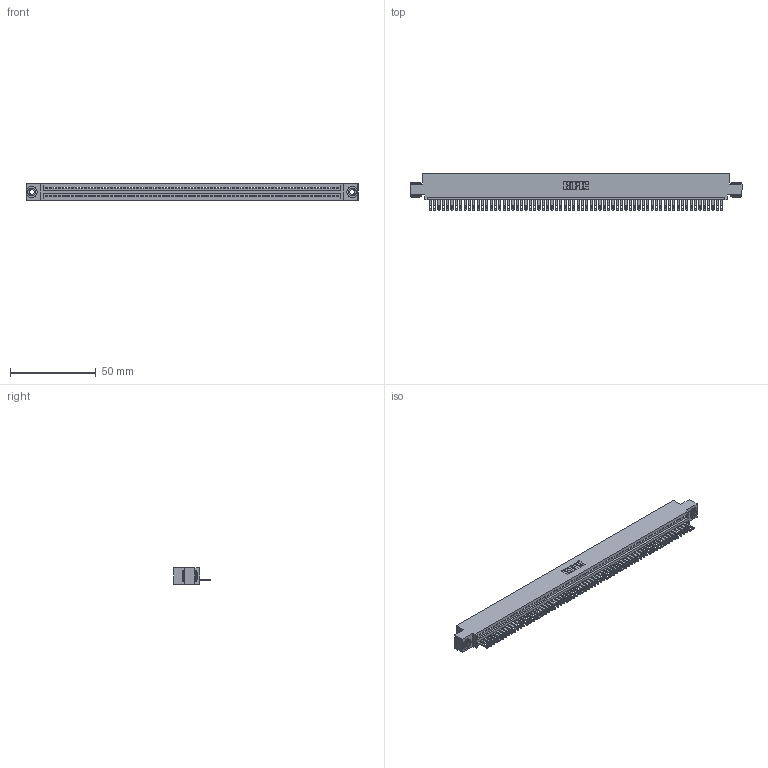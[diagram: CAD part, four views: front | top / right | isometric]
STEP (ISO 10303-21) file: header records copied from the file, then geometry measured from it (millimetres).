
FILE_DESCRIPTION (( 'STEP AP203' ), '1' );
FILE_NAME ('345-068-500-403.STEP', '2019-10-12T03:57:20', ( '' ), ( '' ), 'SwSTEP 2.0', 'SolidWorks 2016', '' );
FILE_SCHEMA (( 'CONFIG_CONTROL_DESIGN' ));
Length unit declared in the file: inch
Products named in the file (4): 345-292-001_345-293-100; 345-068-500-403; 345-250-002_345-250-002-102; 345 Part_0.110 Offset - 0.156 Dia-TH
Assembly tree (71 placements, depth 2):
  345-068-500-403
    345 Part_0.110 Offset - 0.156 Dia-TH
    345-292-001_345-293-100  x68
    345-250-002_345-250-002-102  x2
Bounding box: 193.93 x 21.51 x 9.4 mm (x, y, z)
Volume: 18620.7 mm3; surface area: 25547.6 mm2
Topology: 71 solids, 71 shells, 3840 faces, 11853 edges, 7898 vertices
Faces by surface type: plane 2406, cylinder 1426, cone 8
Entity records: 48390 total; most frequent: CARTESIAN_POINT 8359, ORIENTED_EDGE 8354, DIRECTION 7295, EDGE_CURVE 4177, LINE 3745, VECTOR 3745, VERTEX_POINT 2782, AXIS2_PLACEMENT_3D 1775
